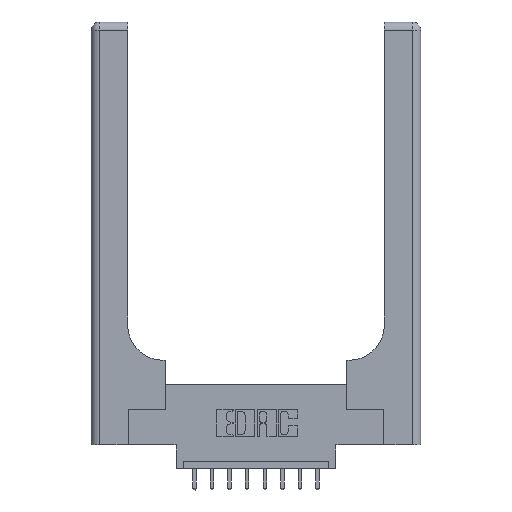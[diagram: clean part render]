
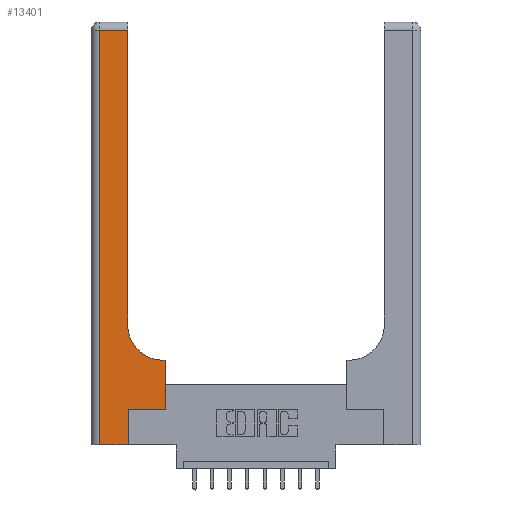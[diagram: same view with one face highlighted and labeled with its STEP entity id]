
A CAD part, top view. The second image highlights one B-rep face of the part: STEP entity #13401.
In plain terms, the highlighted planar face has unit normal (0, 0, 1).
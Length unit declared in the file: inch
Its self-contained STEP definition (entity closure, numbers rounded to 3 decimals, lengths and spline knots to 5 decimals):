
#235 = ORIENTED_EDGE ( 'NONE', *, *, #1291, .T. ) ;
#316 = VERTEX_POINT ( 'NONE', #1345 ) ;
#695 = VERTEX_POINT ( 'NONE', #14309 ) ;
#946 = LINE ( 'NONE', #9265, #1698 ) ;
#1206 = DIRECTION ( 'NONE',  ( 0., -1., 0. ) ) ;
#1291 = EDGE_CURVE ( 'NONE', #695, #9315, #1561, .T. ) ;
#1345 = CARTESIAN_POINT ( 'NONE',  ( 0.528, 0.25, 0.37 ) ) ;
#1548 = CARTESIAN_POINT ( 'NONE',  ( 0.51, 0.6, 0.37 ) ) ;
#1561 = LINE ( 'NONE', #6412, #14670 ) ;
#1698 = VECTOR ( 'NONE', #11738, 39.37008 ) ;
#2106 = CARTESIAN_POINT ( 'NONE',  ( 0.51, 0.85, 0.37 ) ) ;
#2162 = VECTOR ( 'NONE', #3327, 39.37008 ) ;
#2240 = CARTESIAN_POINT ( 'NONE',  ( 0.06, 2.94, 0.37 ) ) ;
#2321 = CARTESIAN_POINT ( 'NONE',  ( 0.06, 3., 0.37 ) ) ;
#2367 = DIRECTION ( 'NONE',  ( 0., 0., -1. ) ) ;
#2473 = CARTESIAN_POINT ( 'NONE',  ( 0., 2.94, 0.37 ) ) ;
#2557 = EDGE_LOOP ( 'NONE', ( #8552, #3990, #5641, #235, #4449, #14764, #10502, #7445, #9016 ) ) ;
#3017 = VECTOR ( 'NONE', #13780, 39.37008 ) ;
#3217 = EDGE_CURVE ( 'NONE', #316, #12210, #946, .T. ) ;
#3286 = VECTOR ( 'NONE', #8667, 39.37008 ) ;
#3327 = DIRECTION ( 'NONE',  ( -1., 0., 0. ) ) ;
#3655 = CARTESIAN_POINT ( 'NONE',  ( 0.26, 2.94, 0.37 ) ) ;
#3990 = ORIENTED_EDGE ( 'NONE', *, *, #10345, .T. ) ;
#4042 = EDGE_CURVE ( 'NONE', #13479, #316, #5666, .T. ) ;
#4236 = CARTESIAN_POINT ( 'NONE',  ( 0.265, 0., 0.37 ) ) ;
#4449 = ORIENTED_EDGE ( 'NONE', *, *, #10031, .T. ) ;
#4625 = FACE_OUTER_BOUND ( 'NONE', #2557, .T. ) ;
#4641 = LINE ( 'NONE', #9240, #2162 ) ;
#4804 = LINE ( 'NONE', #4236, #7145 ) ;
#5238 = CARTESIAN_POINT ( 'NONE',  ( 0.26, 3., 0.37 ) ) ;
#5339 = VERTEX_POINT ( 'NONE', #8381 ) ;
#5641 = ORIENTED_EDGE ( 'NONE', *, *, #11664, .T. ) ;
#5666 = LINE ( 'NONE', #14784, #11376 ) ;
#5767 = CARTESIAN_POINT ( 'NONE',  ( 0.265, 0., 0.37 ) ) ;
#5803 = PLANE ( 'NONE',  #9143 ) ;
#6412 = CARTESIAN_POINT ( 'NONE',  ( 0., 0., 0.37 ) ) ;
#6528 = EDGE_CURVE ( 'NONE', #5339, #9784, #13318, .T. ) ;
#7069 = DIRECTION ( 'NONE',  ( -1., 0., 0. ) ) ;
#7145 = VECTOR ( 'NONE', #12140, 39.37008 ) ;
#7445 = ORIENTED_EDGE ( 'NONE', *, *, #9003, .T. ) ;
#7924 = DIRECTION ( 'NONE',  ( 1., 0., 0. ) ) ;
#8072 = VECTOR ( 'NONE', #1206, 39.37008 ) ;
#8203 = CARTESIAN_POINT ( 'NONE',  ( 0.265, 0.25, 0.37 ) ) ;
#8381 = CARTESIAN_POINT ( 'NONE',  ( 0.26, 0.85, 0.37 ) ) ;
#8552 = ORIENTED_EDGE ( 'NONE', *, *, #6528, .T. ) ;
#8613 = DIRECTION ( 'NONE',  ( 1., 0., 0. ) ) ;
#8667 = DIRECTION ( 'NONE',  ( 0., 1., 0. ) ) ;
#8807 = LINE ( 'NONE', #2321, #8072 ) ;
#8999 = DIRECTION ( 'NONE',  ( 0., 0., -1. ) ) ;
#9003 = EDGE_CURVE ( 'NONE', #12210, #10000, #4641, .T. ) ;
#9016 = ORIENTED_EDGE ( 'NONE', *, *, #12004, .T. ) ;
#9143 = AXIS2_PLACEMENT_3D ( 'NONE', #11577, #2367, #7069 ) ;
#9240 = CARTESIAN_POINT ( 'NONE',  ( 0.26, 0.6, 0.37 ) ) ;
#9265 = CARTESIAN_POINT ( 'NONE',  ( 0.528, 0.25, 0.37 ) ) ;
#9315 = VERTEX_POINT ( 'NONE', #5767 ) ;
#9784 = VERTEX_POINT ( 'NONE', #3655 ) ;
#10000 = VERTEX_POINT ( 'NONE', #1548 ) ;
#10031 = EDGE_CURVE ( 'NONE', #9315, #13479, #4804, .T. ) ;
#10294 = AXIS2_PLACEMENT_3D ( 'NONE', #2106, #8999, #8613 ) ;
#10345 = EDGE_CURVE ( 'NONE', #9784, #11056, #12123, .T. ) ;
#10502 = ORIENTED_EDGE ( 'NONE', *, *, #3217, .T. ) ;
#11056 = VERTEX_POINT ( 'NONE', #2240 ) ;
#11322 = CARTESIAN_POINT ( 'NONE',  ( 0.528, 0.6, 0.37 ) ) ;
#11376 = VECTOR ( 'NONE', #7924, 39.37008 ) ;
#11577 = CARTESIAN_POINT ( 'NONE',  ( 0., 3., 0.37 ) ) ;
#11664 = EDGE_CURVE ( 'NONE', #11056, #695, #8807, .T. ) ;
#11738 = DIRECTION ( 'NONE',  ( 0., 1., 0. ) ) ;
#12004 = EDGE_CURVE ( 'NONE', #10000, #5339, #14743, .T. ) ;
#12123 = LINE ( 'NONE', #2473, #3017 ) ;
#12140 = DIRECTION ( 'NONE',  ( 0., 1., 0. ) ) ;
#12210 = VERTEX_POINT ( 'NONE', #11322 ) ;
#13318 = LINE ( 'NONE', #5238, #3286 ) ;
#13401 = ADVANCED_FACE ( 'NONE', ( #4625 ), #5803, .F. ) ;
#13479 = VERTEX_POINT ( 'NONE', #8203 ) ;
#13780 = DIRECTION ( 'NONE',  ( -1., 0., 0. ) ) ;
#14309 = CARTESIAN_POINT ( 'NONE',  ( 0.06, 0., 0.37 ) ) ;
#14558 = DIRECTION ( 'NONE',  ( 1., 0., 0. ) ) ;
#14670 = VECTOR ( 'NONE', #14558, 39.37008 ) ;
#14743 = CIRCLE ( 'NONE', #10294, 0.25 ) ;
#14764 = ORIENTED_EDGE ( 'NONE', *, *, #4042, .T. ) ;
#14784 = CARTESIAN_POINT ( 'NONE',  ( 0.265, 0.25, 0.37 ) ) ;
